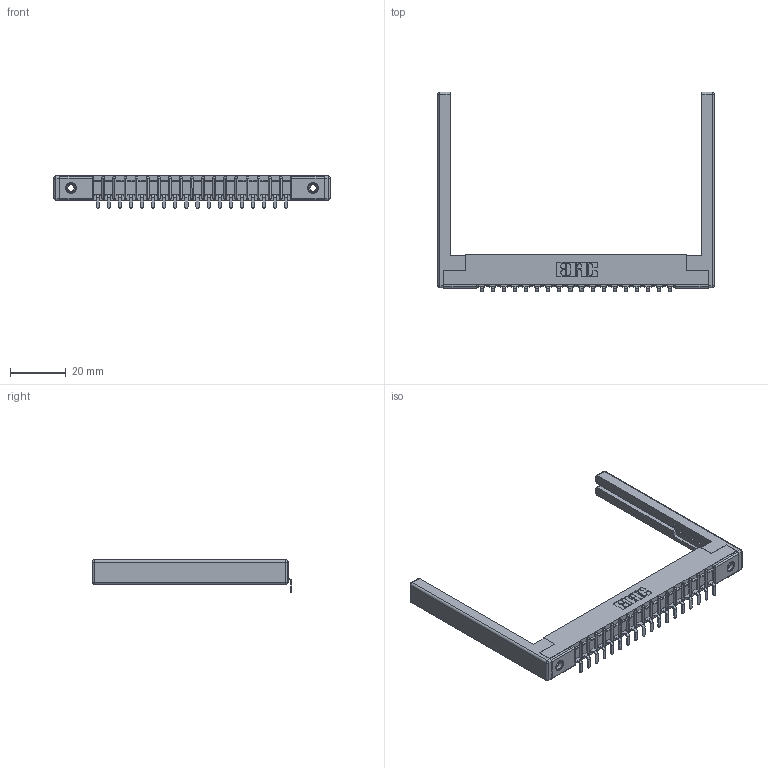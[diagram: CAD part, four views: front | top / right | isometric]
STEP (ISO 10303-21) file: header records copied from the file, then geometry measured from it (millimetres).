
FILE_DESCRIPTION (( 'STEP AP203' ), '1' );
FILE_NAME ('357-018-553-168.STEP', '2019-09-16T21:35:29', ( '' ), ( '' ), 'SwSTEP 2.0', 'SolidWorks 2016', '' );
FILE_SCHEMA (( 'CONFIG_CONTROL_DESIGN' ));
Length unit declared in the file: inch
Products named in the file (5): 307-290-002_553; 357-018-553-168; 307-220-068; 307 Part_.156 Dia Mounting Holes; 345-250-001_345-250-001-102
Assembly tree (23 placements, depth 2):
  357-018-553-168
    307 Part_.156 Dia Mounting Holes
    307-290-002_553  x18
    307-220-068  x2
    345-250-001_345-250-001-102  x2
Bounding box: 98.76 x 71.29 x 11.51 mm (x, y, z)
Volume: 11076.2 mm3; surface area: 15657.7 mm2
Topology: 23 solids, 23 shells, 1695 faces, 5105 edges, 3330 vertices
Faces by surface type: plane 1004, cylinder 629, sphere 46, cone 12, torus 4
Entity records: 22003 total; most frequent: CARTESIAN_POINT 3673, ORIENTED_EDGE 3652, DIRECTION 3598, EDGE_CURVE 1826, LINE 1384, VECTOR 1384, VERTEX_POINT 1182, AXIS2_PLACEMENT_3D 1107
